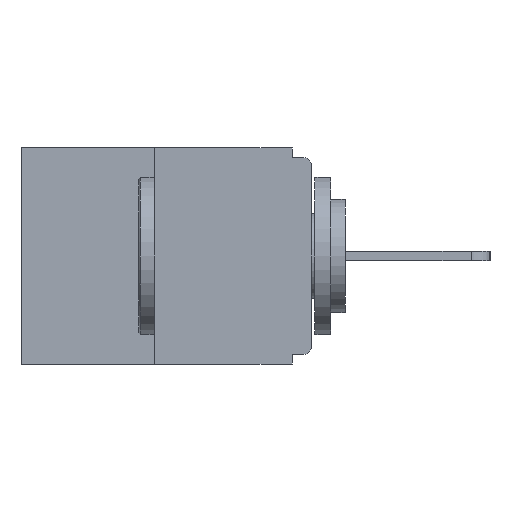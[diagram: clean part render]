
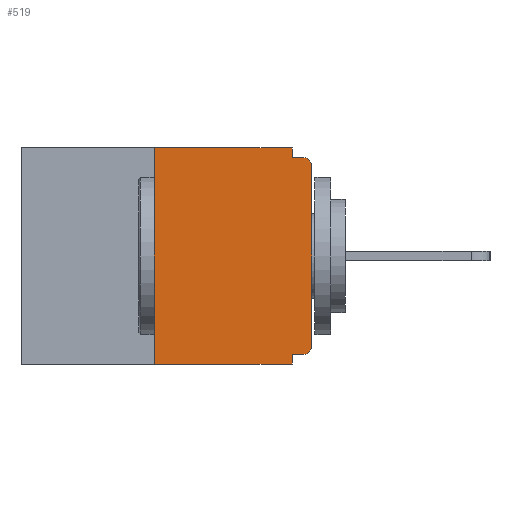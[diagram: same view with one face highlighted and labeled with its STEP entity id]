
A CAD part, left-side view. The second image highlights one B-rep face of the part: STEP entity #519.
In plain terms, the highlighted planar face has unit normal (-1, 0, 0).
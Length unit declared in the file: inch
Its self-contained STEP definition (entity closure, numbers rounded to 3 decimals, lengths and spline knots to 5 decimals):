
#59 = DIRECTION ( 'NONE',  ( 0., 0., 1. ) ) ;
#83 = DIRECTION ( 'NONE',  ( 1., 0., 0. ) ) ;
#133 = ORIENTED_EDGE ( 'NONE', *, *, #7821, .F. ) ;
#412 = LINE ( 'NONE', #9394, #1636 ) ;
#470 = DIRECTION ( 'NONE',  ( 0., 0., -1. ) ) ;
#519 = ADVANCED_FACE ( 'NONE', ( #6288 ), #1435, .F. ) ;
#556 = CARTESIAN_POINT ( 'NONE',  ( 0., 0.015, -0.328 ) ) ;
#591 = ORIENTED_EDGE ( 'NONE', *, *, #14632, .T. ) ;
#867 = CARTESIAN_POINT ( 'NONE',  ( 0., 0.015, -0.015 ) ) ;
#1093 = CARTESIAN_POINT ( 'NONE',  ( 0., 0., 0. ) ) ;
#1135 = CARTESIAN_POINT ( 'NONE',  ( 0., 0.031, -0.015 ) ) ;
#1285 = DIRECTION ( 'NONE',  ( -1., 0., 0. ) ) ;
#1435 = PLANE ( 'NONE',  #15301 ) ;
#1499 = DIRECTION ( 'NONE',  ( 0., 1., 0. ) ) ;
#1636 = VECTOR ( 'NONE', #12869, 39.37008 ) ;
#1669 = VERTEX_POINT ( 'NONE', #13768 ) ;
#1886 = VERTEX_POINT ( 'NONE', #556 ) ;
#2049 = EDGE_CURVE ( 'NONE', #1886, #1669, #6085, .T. ) ;
#2104 = CARTESIAN_POINT ( 'NONE',  ( 0., 0.25, 0. ) ) ;
#2161 = DIRECTION ( 'NONE',  ( 0., 0., 1. ) ) ;
#2376 = AXIS2_PLACEMENT_3D ( 'NONE', #8573, #1285, #9757 ) ;
#2468 = VERTEX_POINT ( 'NONE', #8646 ) ;
#2646 = ORIENTED_EDGE ( 'NONE', *, *, #10910, .F. ) ;
#2814 = EDGE_CURVE ( 'NONE', #1886, #13225, #7904, .T. ) ;
#3545 = ORIENTED_EDGE ( 'NONE', *, *, #14295, .T. ) ;
#3717 = ORIENTED_EDGE ( 'NONE', *, *, #10373, .T. ) ;
#3936 = ORIENTED_EDGE ( 'NONE', *, *, #12755, .F. ) ;
#4000 = EDGE_LOOP ( 'NONE', ( #4047, #133, #591, #2646, #4527, #6116, #3545, #3717, #3936, #4297 ) ) ;
#4047 = ORIENTED_EDGE ( 'NONE', *, *, #7047, .F. ) ;
#4058 = DIRECTION ( 'NONE',  ( 0., 0., -1. ) ) ;
#4297 = ORIENTED_EDGE ( 'NONE', *, *, #4997, .F. ) ;
#4310 = LINE ( 'NONE', #9953, #4472 ) ;
#4472 = VECTOR ( 'NONE', #9683, 39.37008 ) ;
#4527 = ORIENTED_EDGE ( 'NONE', *, *, #2049, .F. ) ;
#4997 = EDGE_CURVE ( 'NONE', #9982, #7413, #7923, .T. ) ;
#5421 = LINE ( 'NONE', #2104, #11285 ) ;
#5755 = VERTEX_POINT ( 'NONE', #867 ) ;
#5980 = DIRECTION ( 'NONE',  ( 0., -1., 0. ) ) ;
#6019 = LINE ( 'NONE', #12762, #14947 ) ;
#6059 = LINE ( 'NONE', #11788, #11890 ) ;
#6085 = LINE ( 'NONE', #14736, #11917 ) ;
#6116 = ORIENTED_EDGE ( 'NONE', *, *, #2814, .T. ) ;
#6288 = FACE_OUTER_BOUND ( 'NONE', #4000, .T. ) ;
#6751 = DIRECTION ( 'NONE',  ( -1., 0., 0. ) ) ;
#7047 = EDGE_CURVE ( 'NONE', #14928, #9982, #4310, .T. ) ;
#7210 = CARTESIAN_POINT ( 'NONE',  ( 0., 0.46, 0. ) ) ;
#7322 = CARTESIAN_POINT ( 'NONE',  ( 0., 0.015, -0.313 ) ) ;
#7413 = VERTEX_POINT ( 'NONE', #1135 ) ;
#7606 = CARTESIAN_POINT ( 'NONE',  ( 0., 0.031, 0. ) ) ;
#7690 = VECTOR ( 'NONE', #59, 39.37008 ) ;
#7821 = EDGE_CURVE ( 'NONE', #11227, #14928, #5421, .T. ) ;
#7871 = AXIS2_PLACEMENT_3D ( 'NONE', #7322, #6751, #470 ) ;
#7904 = CIRCLE ( 'NONE', #7871, 0.015 ) ;
#7923 = LINE ( 'NONE', #7606, #13717 ) ;
#7982 = CARTESIAN_POINT ( 'NONE',  ( 0., 0., -0.313 ) ) ;
#8573 = CARTESIAN_POINT ( 'NONE',  ( 0., 0.015, -0.03 ) ) ;
#8646 = CARTESIAN_POINT ( 'NONE',  ( 0., 0., -0.03 ) ) ;
#8692 = CARTESIAN_POINT ( 'NONE',  ( 0., 0.031, -0.343 ) ) ;
#8862 = CARTESIAN_POINT ( 'NONE',  ( 0., 0.25, -0.343 ) ) ;
#8998 = CARTESIAN_POINT ( 'NONE',  ( 0., 0.031, 0. ) ) ;
#9394 = CARTESIAN_POINT ( 'NONE',  ( 0., 0.031, -0.343 ) ) ;
#9683 = DIRECTION ( 'NONE',  ( 0., -1., 0. ) ) ;
#9757 = DIRECTION ( 'NONE',  ( 0., 0., -1. ) ) ;
#9840 = VERTEX_POINT ( 'NONE', #8692 ) ;
#9953 = CARTESIAN_POINT ( 'NONE',  ( 0., 0.46, 0. ) ) ;
#9982 = VERTEX_POINT ( 'NONE', #8998 ) ;
#10373 = EDGE_CURVE ( 'NONE', #2468, #5755, #11574, .T. ) ;
#10910 = EDGE_CURVE ( 'NONE', #1669, #9840, #412, .T. ) ;
#11227 = VERTEX_POINT ( 'NONE', #8862 ) ;
#11285 = VECTOR ( 'NONE', #2161, 39.37008 ) ;
#11574 = CIRCLE ( 'NONE', #2376, 0.015 ) ;
#11788 = CARTESIAN_POINT ( 'NONE',  ( 0., 0., -0.015 ) ) ;
#11890 = VECTOR ( 'NONE', #5980, 39.37008 ) ;
#11917 = VECTOR ( 'NONE', #1499, 39.37008 ) ;
#11926 = DIRECTION ( 'NONE',  ( 0., 0., -1. ) ) ;
#12755 = EDGE_CURVE ( 'NONE', #7413, #5755, #6059, .T. ) ;
#12762 = CARTESIAN_POINT ( 'NONE',  ( 0., 0.46, -0.343 ) ) ;
#12869 = DIRECTION ( 'NONE',  ( 0., 0., -1. ) ) ;
#13225 = VERTEX_POINT ( 'NONE', #7982 ) ;
#13717 = VECTOR ( 'NONE', #4058, 39.37008 ) ;
#13768 = CARTESIAN_POINT ( 'NONE',  ( 0., 0.031, -0.328 ) ) ;
#13853 = LINE ( 'NONE', #1093, #7690 ) ;
#14295 = EDGE_CURVE ( 'NONE', #13225, #2468, #13853, .T. ) ;
#14467 = CARTESIAN_POINT ( 'NONE',  ( 0., 0.25, 0. ) ) ;
#14632 = EDGE_CURVE ( 'NONE', #11227, #9840, #6019, .T. ) ;
#14736 = CARTESIAN_POINT ( 'NONE',  ( 0., 0., -0.328 ) ) ;
#14928 = VERTEX_POINT ( 'NONE', #14467 ) ;
#14947 = VECTOR ( 'NONE', #15089, 39.37008 ) ;
#15089 = DIRECTION ( 'NONE',  ( 0., -1., 0. ) ) ;
#15301 = AXIS2_PLACEMENT_3D ( 'NONE', #7210, #83, #11926 ) ;
